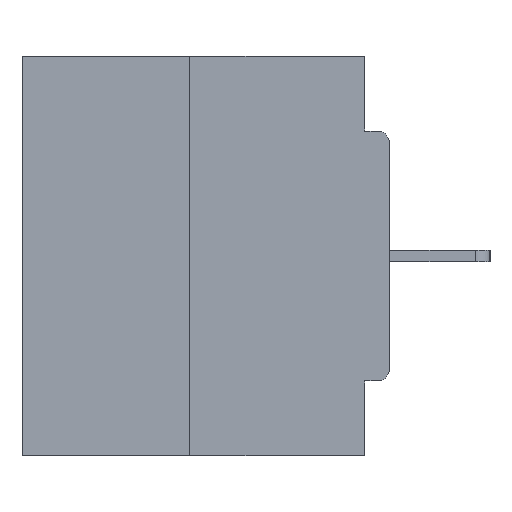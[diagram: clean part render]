
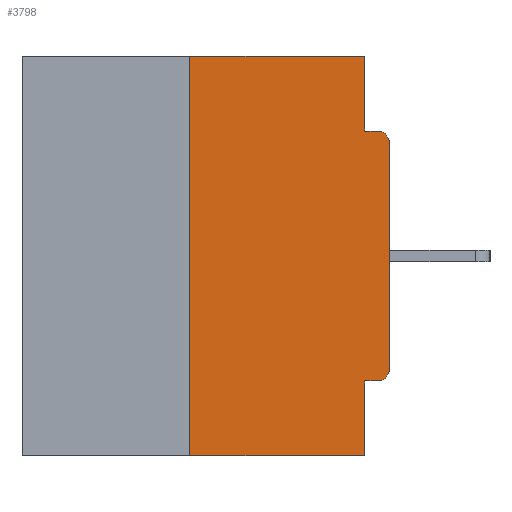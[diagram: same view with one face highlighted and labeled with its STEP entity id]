
A CAD part, left-side view. The second image highlights one B-rep face of the part: STEP entity #3798.
In plain terms, the highlighted planar face has unit normal (-1, 0, 0).
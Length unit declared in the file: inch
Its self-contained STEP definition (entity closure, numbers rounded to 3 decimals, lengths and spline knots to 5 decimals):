
#357 = CARTESIAN_POINT ( 'NONE',  ( 0., 0., -0.1085 ) ) ;
#497 = CIRCLE ( 'NONE', #18185, 0.015 ) ;
#576 = DIRECTION ( 'NONE',  ( 0., 1., 0. ) ) ;
#1324 = FACE_OUTER_BOUND ( 'NONE', #12313, .T. ) ;
#1591 = VERTEX_POINT ( 'NONE', #12258 ) ;
#1749 = CARTESIAN_POINT ( 'NONE',  ( 0., 0.015, -0.4065 ) ) ;
#2236 = CARTESIAN_POINT ( 'NONE',  ( 0., 0.031, 0. ) ) ;
#2980 = EDGE_CURVE ( 'NONE', #10640, #14127, #14993, .T. ) ;
#3241 = CARTESIAN_POINT ( 'NONE',  ( 0., 0.46, -0.5 ) ) ;
#3362 = CARTESIAN_POINT ( 'NONE',  ( 0., 0.015, -0.0935 ) ) ;
#3495 = DIRECTION ( 'NONE',  ( 0., -1., 0. ) ) ;
#3514 = CARTESIAN_POINT ( 'NONE',  ( 0., 0.031, -0.5 ) ) ;
#3798 = ADVANCED_FACE ( 'NONE', ( #1324 ), #20500, .F. ) ;
#3876 = DIRECTION ( 'NONE',  ( -1., 0., 0. ) ) ;
#4774 = VECTOR ( 'NONE', #576, 39.37008 ) ;
#5124 = VECTOR ( 'NONE', #25397, 39.37008 ) ;
#5560 = LINE ( 'NONE', #30100, #4774 ) ;
#5855 = LINE ( 'NONE', #16262, #31081 ) ;
#7235 = LINE ( 'NONE', #15037, #17944 ) ;
#7262 = CARTESIAN_POINT ( 'NONE',  ( 0., 0.46, 0. ) ) ;
#7419 = EDGE_CURVE ( 'NONE', #1591, #16115, #27378, .T. ) ;
#7506 = VERTEX_POINT ( 'NONE', #1749 ) ;
#7728 = ORIENTED_EDGE ( 'NONE', *, *, #31701, .F. ) ;
#8455 = VECTOR ( 'NONE', #8812, 39.37008 ) ;
#8469 = ORIENTED_EDGE ( 'NONE', *, *, #7419, .T. ) ;
#8488 = CARTESIAN_POINT ( 'NONE',  ( 0., 0.46, 0. ) ) ;
#8589 = EDGE_CURVE ( 'NONE', #7506, #14308, #497, .T. ) ;
#8812 = DIRECTION ( 'NONE',  ( 0., 0., -1. ) ) ;
#8953 = DIRECTION ( 'NONE',  ( 0., -1., 0. ) ) ;
#9134 = DIRECTION ( 'NONE',  ( 0., 0., -1. ) ) ;
#9243 = DIRECTION ( 'NONE',  ( 1., 0., 0. ) ) ;
#9423 = VERTEX_POINT ( 'NONE', #357 ) ;
#9451 = AXIS2_PLACEMENT_3D ( 'NONE', #8488, #9243, #9134 ) ;
#9824 = CARTESIAN_POINT ( 'NONE',  ( 0., 0., -0.3915 ) ) ;
#10016 = ORIENTED_EDGE ( 'NONE', *, *, #23638, .F. ) ;
#10640 = VERTEX_POINT ( 'NONE', #2236 ) ;
#11547 = ORIENTED_EDGE ( 'NONE', *, *, #15791, .T. ) ;
#11993 = CIRCLE ( 'NONE', #20395, 0.015 ) ;
#12258 = CARTESIAN_POINT ( 'NONE',  ( 0., 0.25, -0.5 ) ) ;
#12313 = EDGE_LOOP ( 'NONE', ( #7728, #27266, #8469, #15771, #10016, #23080, #30276, #11547, #26124, #20385 ) ) ;
#13095 = CARTESIAN_POINT ( 'NONE',  ( 0., 0.25, 0. ) ) ;
#13517 = LINE ( 'NONE', #7262, #31453 ) ;
#14127 = VERTEX_POINT ( 'NONE', #21299 ) ;
#14308 = VERTEX_POINT ( 'NONE', #9824 ) ;
#14993 = LINE ( 'NONE', #31640, #8455 ) ;
#15037 = CARTESIAN_POINT ( 'NONE',  ( 0., 0., 0. ) ) ;
#15123 = CARTESIAN_POINT ( 'NONE',  ( 0., 0.25, 0. ) ) ;
#15771 = ORIENTED_EDGE ( 'NONE', *, *, #21160, .F. ) ;
#15791 = EDGE_CURVE ( 'NONE', #9423, #26956, #11993, .T. ) ;
#16115 = VERTEX_POINT ( 'NONE', #17439 ) ;
#16262 = CARTESIAN_POINT ( 'NONE',  ( 0., 0., -0.0935 ) ) ;
#17439 = CARTESIAN_POINT ( 'NONE',  ( 0., 0.031, -0.5 ) ) ;
#17944 = VECTOR ( 'NONE', #29645, 39.37008 ) ;
#17969 = LINE ( 'NONE', #3514, #24503 ) ;
#18185 = AXIS2_PLACEMENT_3D ( 'NONE', #23695, #23649, #23612 ) ;
#18636 = CARTESIAN_POINT ( 'NONE',  ( 0., 0.015, -0.1085 ) ) ;
#19255 = VERTEX_POINT ( 'NONE', #23548 ) ;
#20385 = ORIENTED_EDGE ( 'NONE', *, *, #2980, .F. ) ;
#20395 = AXIS2_PLACEMENT_3D ( 'NONE', #18636, #3876, #21108 ) ;
#20500 = PLANE ( 'NONE',  #9451 ) ;
#20770 = DIRECTION ( 'NONE',  ( 0., 0., -1. ) ) ;
#21108 = DIRECTION ( 'NONE',  ( 0., 0., -1. ) ) ;
#21160 = EDGE_CURVE ( 'NONE', #19255, #16115, #17969, .T. ) ;
#21299 = CARTESIAN_POINT ( 'NONE',  ( 0., 0.031, -0.0935 ) ) ;
#22230 = VERTEX_POINT ( 'NONE', #15123 ) ;
#23080 = ORIENTED_EDGE ( 'NONE', *, *, #8589, .T. ) ;
#23548 = CARTESIAN_POINT ( 'NONE',  ( 0., 0.031, -0.4065 ) ) ;
#23612 = DIRECTION ( 'NONE',  ( 0., 0., -1. ) ) ;
#23638 = EDGE_CURVE ( 'NONE', #7506, #19255, #5560, .T. ) ;
#23649 = DIRECTION ( 'NONE',  ( -1., 0., 0. ) ) ;
#23695 = CARTESIAN_POINT ( 'NONE',  ( 0., 0.015, -0.3915 ) ) ;
#24267 = EDGE_CURVE ( 'NONE', #1591, #22230, #24707, .T. ) ;
#24503 = VECTOR ( 'NONE', #20770, 39.37008 ) ;
#24707 = LINE ( 'NONE', #13095, #5124 ) ;
#25397 = DIRECTION ( 'NONE',  ( 0., 0., 1. ) ) ;
#26124 = ORIENTED_EDGE ( 'NONE', *, *, #31510, .F. ) ;
#26615 = VECTOR ( 'NONE', #3495, 39.37008 ) ;
#26760 = DIRECTION ( 'NONE',  ( 0., -1., 0. ) ) ;
#26956 = VERTEX_POINT ( 'NONE', #3362 ) ;
#27266 = ORIENTED_EDGE ( 'NONE', *, *, #24267, .F. ) ;
#27378 = LINE ( 'NONE', #3241, #26615 ) ;
#28158 = EDGE_CURVE ( 'NONE', #14308, #9423, #7235, .T. ) ;
#29645 = DIRECTION ( 'NONE',  ( 0., 0., 1. ) ) ;
#30100 = CARTESIAN_POINT ( 'NONE',  ( 0., 0., -0.4065 ) ) ;
#30276 = ORIENTED_EDGE ( 'NONE', *, *, #28158, .T. ) ;
#31081 = VECTOR ( 'NONE', #8953, 39.37008 ) ;
#31453 = VECTOR ( 'NONE', #26760, 39.37008 ) ;
#31510 = EDGE_CURVE ( 'NONE', #14127, #26956, #5855, .T. ) ;
#31640 = CARTESIAN_POINT ( 'NONE',  ( 0., 0.031, 0. ) ) ;
#31701 = EDGE_CURVE ( 'NONE', #22230, #10640, #13517, .T. ) ;
